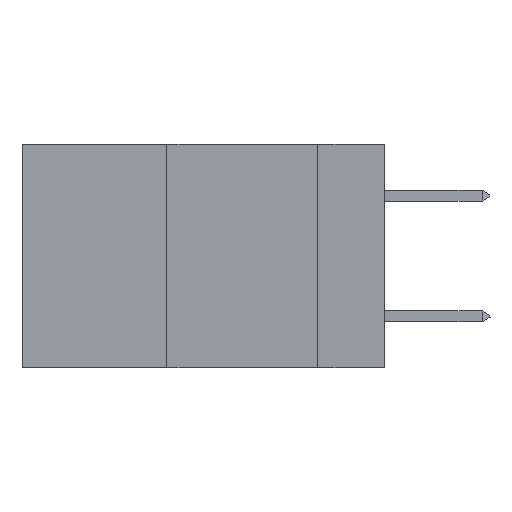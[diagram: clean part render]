
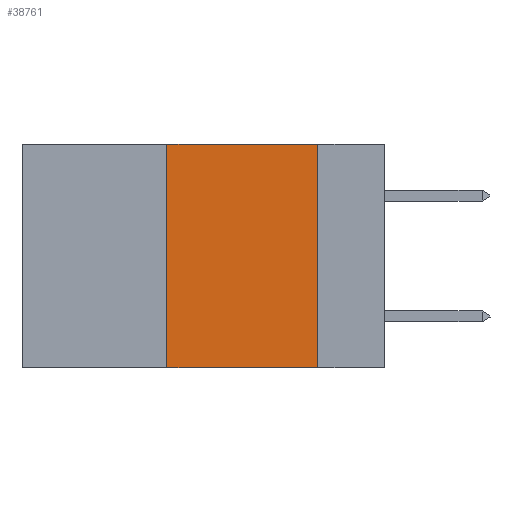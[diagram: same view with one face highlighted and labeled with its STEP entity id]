
A CAD part, left-side view. The second image highlights one B-rep face of the part: STEP entity #38761.
In plain terms, the highlighted planar face has unit normal (-1, 0, 0).
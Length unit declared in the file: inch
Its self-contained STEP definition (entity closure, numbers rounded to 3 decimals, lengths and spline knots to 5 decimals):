
#168 = LINE ( 'NONE', #36766, #23265 ) ;
#394 = CARTESIAN_POINT ( 'NONE',  ( 0., 0.6, 0. ) ) ;
#875 = CARTESIAN_POINT ( 'NONE',  ( 0., 0.11, 0. ) ) ;
#1251 = EDGE_LOOP ( 'NONE', ( #12120, #13525, #42177, #8064 ) ) ;
#4401 = EDGE_CURVE ( 'NONE', #17537, #19503, #34923, .T. ) ;
#4698 = CARTESIAN_POINT ( 'NONE',  ( 0., 0.11, 0. ) ) ;
#6887 = DIRECTION ( 'NONE',  ( 0., 0., -1. ) ) ;
#7033 = VERTEX_POINT ( 'NONE', #875 ) ;
#7316 = FACE_OUTER_BOUND ( 'NONE', #1251, .T. ) ;
#8064 = ORIENTED_EDGE ( 'NONE', *, *, #4401, .T. ) ;
#11604 = LINE ( 'NONE', #4698, #13022 ) ;
#12120 = ORIENTED_EDGE ( 'NONE', *, *, #23093, .F. ) ;
#12994 = DIRECTION ( 'NONE',  ( 0., -1., 0. ) ) ;
#13022 = VECTOR ( 'NONE', #32576, 39.37008 ) ;
#13216 = CARTESIAN_POINT ( 'NONE',  ( 0., 0.6, 0. ) ) ;
#13525 = ORIENTED_EDGE ( 'NONE', *, *, #14600, .F. ) ;
#14600 = EDGE_CURVE ( 'NONE', #15206, #7033, #43760, .T. ) ;
#15206 = VERTEX_POINT ( 'NONE', #27818 ) ;
#17312 = VECTOR ( 'NONE', #38717, 39.37008 ) ;
#17537 = VERTEX_POINT ( 'NONE', #34543 ) ;
#19503 = VERTEX_POINT ( 'NONE', #21559 ) ;
#21224 = AXIS2_PLACEMENT_3D ( 'NONE', #394, #41217, #6887 ) ;
#21559 = CARTESIAN_POINT ( 'NONE',  ( 0., 0.11, -0.37 ) ) ;
#22520 = CARTESIAN_POINT ( 'NONE',  ( 0., 0.6, -0.37 ) ) ;
#23093 = EDGE_CURVE ( 'NONE', #7033, #19503, #11604, .T. ) ;
#23265 = VECTOR ( 'NONE', #37642, 39.37008 ) ;
#26386 = VECTOR ( 'NONE', #12994, 39.37008 ) ;
#27818 = CARTESIAN_POINT ( 'NONE',  ( 0., 0.36, 0. ) ) ;
#32576 = DIRECTION ( 'NONE',  ( 0., 0., -1. ) ) ;
#34543 = CARTESIAN_POINT ( 'NONE',  ( 0., 0.36, -0.37 ) ) ;
#34923 = LINE ( 'NONE', #22520, #17312 ) ;
#36766 = CARTESIAN_POINT ( 'NONE',  ( 0., 0.36, 0. ) ) ;
#37508 = EDGE_CURVE ( 'NONE', #17537, #15206, #168, .T. ) ;
#37642 = DIRECTION ( 'NONE',  ( 0., 0., 1. ) ) ;
#38717 = DIRECTION ( 'NONE',  ( 0., -1., 0. ) ) ;
#38761 = ADVANCED_FACE ( 'NONE', ( #7316 ), #40996, .F. ) ;
#40996 = PLANE ( 'NONE',  #21224 ) ;
#41217 = DIRECTION ( 'NONE',  ( 1., 0., 0. ) ) ;
#42177 = ORIENTED_EDGE ( 'NONE', *, *, #37508, .F. ) ;
#43760 = LINE ( 'NONE', #13216, #26386 ) ;
